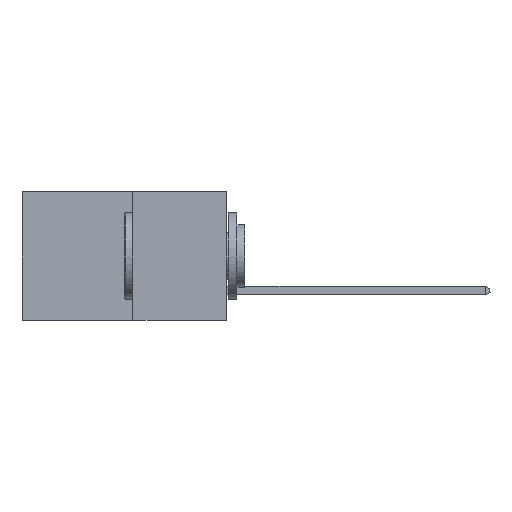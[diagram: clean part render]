
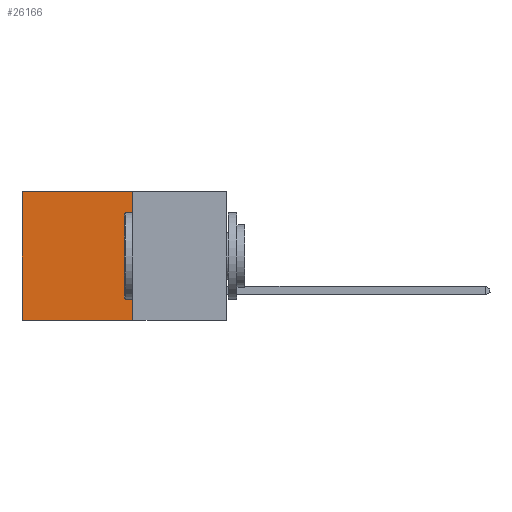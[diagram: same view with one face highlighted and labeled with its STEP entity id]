
A CAD part, left-side view. The second image highlights one B-rep face of the part: STEP entity #26166.
In plain terms, the highlighted planar face has unit normal (-1, 0, 0).
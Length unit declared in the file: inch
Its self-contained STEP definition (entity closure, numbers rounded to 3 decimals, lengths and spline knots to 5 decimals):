
#149 = EDGE_CURVE ( 'NONE', #8626, #15359, #13678, .T. ) ;
#1008 = CARTESIAN_POINT ( 'NONE',  ( 0.277, 0.59, -0.37 ) ) ;
#1296 = FACE_OUTER_BOUND ( 'NONE', #26611, .T. ) ;
#1374 = DIRECTION ( 'NONE',  ( 0., 0., -1. ) ) ;
#1640 = AXIS2_PLACEMENT_3D ( 'NONE', #14483, #6137, #18652 ) ;
#1982 = EDGE_CURVE ( 'NONE', #11389, #18745, #16657, .T. ) ;
#2418 = CARTESIAN_POINT ( 'NONE',  ( 0.277, 0.27, -0.37 ) ) ;
#2790 = LINE ( 'NONE', #26294, #13869 ) ;
#4559 = EDGE_CURVE ( 'NONE', #8626, #11389, #15849, .T. ) ;
#4795 = VECTOR ( 'NONE', #13258, 39.37008 ) ;
#6137 = DIRECTION ( 'NONE',  ( 1., 0., 0. ) ) ;
#6296 = CARTESIAN_POINT ( 'NONE',  ( 0.277, 0.59, 0. ) ) ;
#8626 = VERTEX_POINT ( 'NONE', #23470 ) ;
#9468 = ORIENTED_EDGE ( 'NONE', *, *, #4559, .F. ) ;
#9575 = ORIENTED_EDGE ( 'NONE', *, *, #1982, .F. ) ;
#11389 = VERTEX_POINT ( 'NONE', #21984 ) ;
#13013 = VECTOR ( 'NONE', #19694, 39.37008 ) ;
#13189 = ORIENTED_EDGE ( 'NONE', *, *, #18865, .T. ) ;
#13258 = DIRECTION ( 'NONE',  ( 0., 0., -1. ) ) ;
#13486 = ORIENTED_EDGE ( 'NONE', *, *, #149, .T. ) ;
#13678 = LINE ( 'NONE', #19249, #13013 ) ;
#13869 = VECTOR ( 'NONE', #1374, 39.37008 ) ;
#13913 = CARTESIAN_POINT ( 'NONE',  ( 0.277, 0.27, -0.37 ) ) ;
#14483 = CARTESIAN_POINT ( 'NONE',  ( 0.277, 0.27, -0.37 ) ) ;
#15359 = VERTEX_POINT ( 'NONE', #6296 ) ;
#15849 = LINE ( 'NONE', #13913, #4795 ) ;
#16556 = PLANE ( 'NONE',  #1640 ) ;
#16657 = LINE ( 'NONE', #2418, #21608 ) ;
#18652 = DIRECTION ( 'NONE',  ( 0., 0., -1. ) ) ;
#18745 = VERTEX_POINT ( 'NONE', #1008 ) ;
#18865 = EDGE_CURVE ( 'NONE', #15359, #18745, #2790, .T. ) ;
#19249 = CARTESIAN_POINT ( 'NONE',  ( 0.277, 0.27, 0. ) ) ;
#19694 = DIRECTION ( 'NONE',  ( 0., 1., 0. ) ) ;
#21608 = VECTOR ( 'NONE', #21996, 39.37008 ) ;
#21984 = CARTESIAN_POINT ( 'NONE',  ( 0.277, 0.27, -0.37 ) ) ;
#21996 = DIRECTION ( 'NONE',  ( 0., 1., 0. ) ) ;
#23470 = CARTESIAN_POINT ( 'NONE',  ( 0.277, 0.27, 0. ) ) ;
#26166 = ADVANCED_FACE ( 'NONE', ( #1296 ), #16556, .F. ) ;
#26294 = CARTESIAN_POINT ( 'NONE',  ( 0.277, 0.59, -0.37 ) ) ;
#26611 = EDGE_LOOP ( 'NONE', ( #13189, #9575, #9468, #13486 ) ) ;
